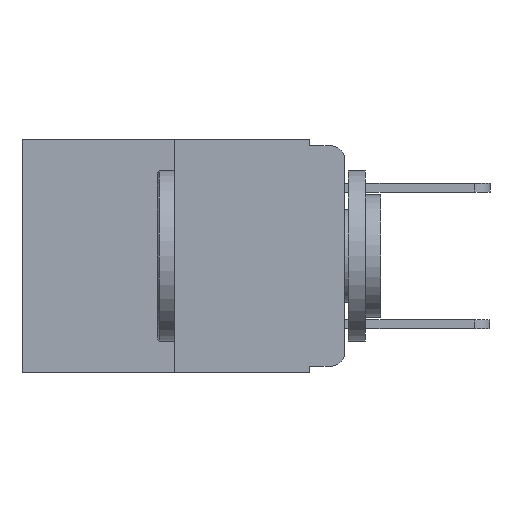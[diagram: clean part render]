
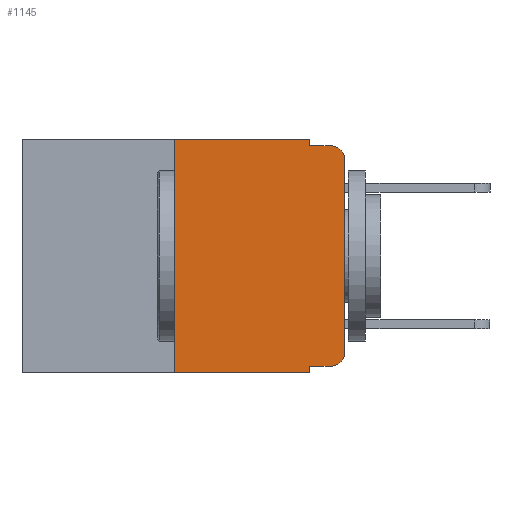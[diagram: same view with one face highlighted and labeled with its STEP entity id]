
A CAD part, left-side view. The second image highlights one B-rep face of the part: STEP entity #1145.
In plain terms, the highlighted planar face has unit normal (-1, 0, 0).
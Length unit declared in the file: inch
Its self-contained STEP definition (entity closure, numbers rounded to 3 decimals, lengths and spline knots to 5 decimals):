
#1 = DIRECTION ( 'NONE',  ( 0., -1., 0. ) ) ;
#260 = ORIENTED_EDGE ( 'NONE', *, *, #9224, .F. ) ;
#303 = ORIENTED_EDGE ( 'NONE', *, *, #10545, .F. ) ;
#327 = DIRECTION ( 'NONE',  ( 0., -1., 0. ) ) ;
#355 = VERTEX_POINT ( 'NONE', #10273 ) ;
#367 = EDGE_CURVE ( 'NONE', #8114, #6384, #7365, .T. ) ;
#417 = VERTEX_POINT ( 'NONE', #8513 ) ;
#486 = EDGE_CURVE ( 'NONE', #2238, #3248, #3629, .T. ) ;
#737 = VECTOR ( 'NONE', #4276, 39.37008 ) ;
#795 = VERTEX_POINT ( 'NONE', #2315 ) ;
#814 = ORIENTED_EDGE ( 'NONE', *, *, #2879, .T. ) ;
#898 = CARTESIAN_POINT ( 'NONE',  ( 0., 0.051, -0.333 ) ) ;
#958 = ORIENTED_EDGE ( 'NONE', *, *, #367, .F. ) ;
#1043 = CARTESIAN_POINT ( 'NONE',  ( 0., 0., -0.03 ) ) ;
#1145 = ADVANCED_FACE ( 'NONE', ( #10436 ), #6763, .F. ) ;
#1219 = CARTESIAN_POINT ( 'NONE',  ( 0., 0.051, 0. ) ) ;
#1232 = CARTESIAN_POINT ( 'NONE',  ( 0., 0.473, 0. ) ) ;
#1563 = VERTEX_POINT ( 'NONE', #4065 ) ;
#1619 = DIRECTION ( 'NONE',  ( -1., 0., 0. ) ) ;
#1630 = CARTESIAN_POINT ( 'NONE',  ( 0., 0.051, 0. ) ) ;
#2128 = ORIENTED_EDGE ( 'NONE', *, *, #10657, .T. ) ;
#2138 = ORIENTED_EDGE ( 'NONE', *, *, #2612, .T. ) ;
#2155 = CARTESIAN_POINT ( 'NONE',  ( 0., 0., 0. ) ) ;
#2238 = VERTEX_POINT ( 'NONE', #11456 ) ;
#2248 = LINE ( 'NONE', #1630, #9788 ) ;
#2315 = CARTESIAN_POINT ( 'NONE',  ( 0., 0.25, -0.343 ) ) ;
#2612 = EDGE_CURVE ( 'NONE', #355, #9341, #4179, .T. ) ;
#2789 = VERTEX_POINT ( 'NONE', #7720 ) ;
#2843 = EDGE_LOOP ( 'NONE', ( #2138, #3081, #10582, #12027, #260, #303, #814, #958, #2128, #3914 ) ) ;
#2852 = CARTESIAN_POINT ( 'NONE',  ( 0., 0.02, -0.03 ) ) ;
#2879 = EDGE_CURVE ( 'NONE', #795, #6384, #8497, .T. ) ;
#2975 = EDGE_CURVE ( 'NONE', #2789, #2238, #2248, .T. ) ;
#3081 = ORIENTED_EDGE ( 'NONE', *, *, #12318, .T. ) ;
#3248 = VERTEX_POINT ( 'NONE', #7096 ) ;
#3328 = VECTOR ( 'NONE', #1, 39.37008 ) ;
#3376 = AXIS2_PLACEMENT_3D ( 'NONE', #2852, #9654, #3944 ) ;
#3629 = LINE ( 'NONE', #12568, #5929 ) ;
#3785 = LINE ( 'NONE', #4852, #8605 ) ;
#3914 = ORIENTED_EDGE ( 'NONE', *, *, #6884, .T. ) ;
#3944 = DIRECTION ( 'NONE',  ( 0., 0., -1. ) ) ;
#4065 = CARTESIAN_POINT ( 'NONE',  ( 0., 0.02, -0.333 ) ) ;
#4179 = LINE ( 'NONE', #2155, #737 ) ;
#4276 = DIRECTION ( 'NONE',  ( 0., 0., 1. ) ) ;
#4309 = DIRECTION ( 'NONE',  ( 0., 0., -1. ) ) ;
#4852 = CARTESIAN_POINT ( 'NONE',  ( 0., 0.473, 0. ) ) ;
#5215 = VECTOR ( 'NONE', #4309, 39.37008 ) ;
#5929 = VECTOR ( 'NONE', #12675, 39.37008 ) ;
#6245 = AXIS2_PLACEMENT_3D ( 'NONE', #7704, #1619, #8710 ) ;
#6384 = VERTEX_POINT ( 'NONE', #12310 ) ;
#6763 = PLANE ( 'NONE',  #9048 ) ;
#6884 = EDGE_CURVE ( 'NONE', #1563, #355, #6962, .T. ) ;
#6895 = CARTESIAN_POINT ( 'NONE',  ( 0., 0.051, -0.333 ) ) ;
#6940 = CARTESIAN_POINT ( 'NONE',  ( 0., 0.25, 0. ) ) ;
#6962 = CIRCLE ( 'NONE', #6245, 0.02 ) ;
#7096 = CARTESIAN_POINT ( 'NONE',  ( 0., 0.02, -0.01 ) ) ;
#7365 = LINE ( 'NONE', #1219, #5215 ) ;
#7437 = DIRECTION ( 'NONE',  ( 1., 0., 0. ) ) ;
#7704 = CARTESIAN_POINT ( 'NONE',  ( 0., 0.02, -0.313 ) ) ;
#7720 = CARTESIAN_POINT ( 'NONE',  ( 0., 0.051, 0. ) ) ;
#7906 = CIRCLE ( 'NONE', #3376, 0.02 ) ;
#7962 = DIRECTION ( 'NONE',  ( 0., 0., 1. ) ) ;
#8114 = VERTEX_POINT ( 'NONE', #6895 ) ;
#8129 = DIRECTION ( 'NONE',  ( 0., -1., 0. ) ) ;
#8263 = VECTOR ( 'NONE', #7962, 39.37008 ) ;
#8427 = DIRECTION ( 'NONE',  ( 0., 0., -1. ) ) ;
#8497 = LINE ( 'NONE', #12579, #3328 ) ;
#8513 = CARTESIAN_POINT ( 'NONE',  ( 0., 0.25, 0. ) ) ;
#8605 = VECTOR ( 'NONE', #327, 39.37008 ) ;
#8710 = DIRECTION ( 'NONE',  ( 0., 0., -1. ) ) ;
#9048 = AXIS2_PLACEMENT_3D ( 'NONE', #1232, #7437, #9863 ) ;
#9224 = EDGE_CURVE ( 'NONE', #417, #2789, #3785, .T. ) ;
#9341 = VERTEX_POINT ( 'NONE', #1043 ) ;
#9654 = DIRECTION ( 'NONE',  ( -1., 0., 0. ) ) ;
#9788 = VECTOR ( 'NONE', #8427, 39.37008 ) ;
#9863 = DIRECTION ( 'NONE',  ( 0., 0., -1. ) ) ;
#10273 = CARTESIAN_POINT ( 'NONE',  ( 0., 0., -0.313 ) ) ;
#10436 = FACE_OUTER_BOUND ( 'NONE', #2843, .T. ) ;
#10545 = EDGE_CURVE ( 'NONE', #795, #417, #10720, .T. ) ;
#10582 = ORIENTED_EDGE ( 'NONE', *, *, #486, .F. ) ;
#10657 = EDGE_CURVE ( 'NONE', #8114, #1563, #12161, .T. ) ;
#10720 = LINE ( 'NONE', #6940, #8263 ) ;
#11456 = CARTESIAN_POINT ( 'NONE',  ( 0., 0.051, -0.01 ) ) ;
#11906 = VECTOR ( 'NONE', #8129, 39.37008 ) ;
#12027 = ORIENTED_EDGE ( 'NONE', *, *, #2975, .F. ) ;
#12161 = LINE ( 'NONE', #898, #11906 ) ;
#12310 = CARTESIAN_POINT ( 'NONE',  ( 0., 0.051, -0.343 ) ) ;
#12318 = EDGE_CURVE ( 'NONE', #9341, #3248, #7906, .T. ) ;
#12568 = CARTESIAN_POINT ( 'NONE',  ( 0., 0.051, -0.01 ) ) ;
#12579 = CARTESIAN_POINT ( 'NONE',  ( 0., 0.473, -0.343 ) ) ;
#12675 = DIRECTION ( 'NONE',  ( 0., -1., 0. ) ) ;
